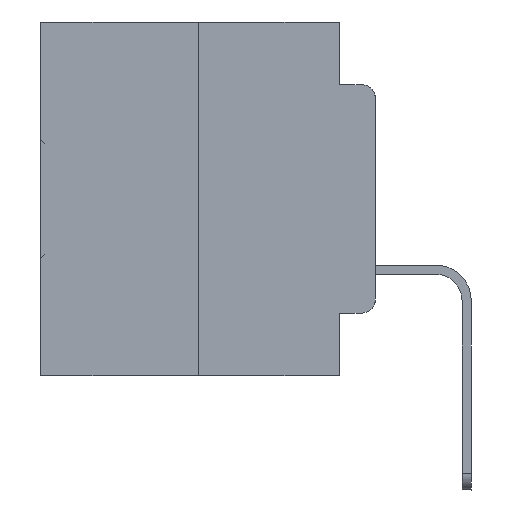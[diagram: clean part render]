
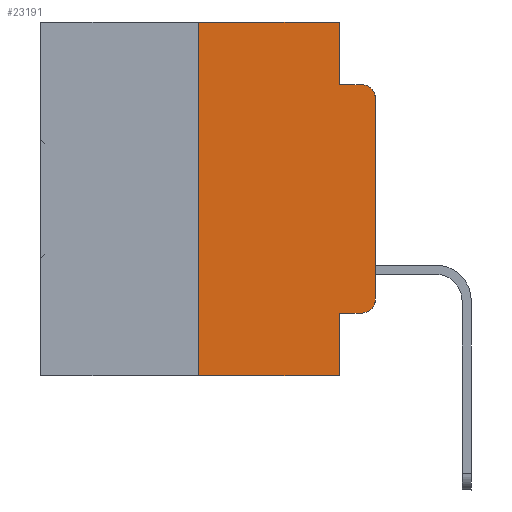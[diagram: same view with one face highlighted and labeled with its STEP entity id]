
A CAD part, left-side view. The second image highlights one B-rep face of the part: STEP entity #23191.
In plain terms, the highlighted planar face has unit normal (-1, 0, 0).
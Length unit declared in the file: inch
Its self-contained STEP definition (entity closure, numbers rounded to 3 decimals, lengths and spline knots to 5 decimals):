
#447 = LINE ( 'NONE', #4120, #23621 ) ;
#589 = EDGE_CURVE ( 'NONE', #5227, #32426, #15324, .T. ) ;
#805 = ORIENTED_EDGE ( 'NONE', *, *, #589, .T. ) ;
#882 = CARTESIAN_POINT ( 'NONE',  ( 0., 0.25, 0. ) ) ;
#2688 = DIRECTION ( 'NONE',  ( 0., 0., -1. ) ) ;
#2972 = FACE_OUTER_BOUND ( 'NONE', #23534, .T. ) ;
#3366 = CARTESIAN_POINT ( 'NONE',  ( 0., 0.02, -0.0885 ) ) ;
#3687 = LINE ( 'NONE', #19408, #24400 ) ;
#3835 = DIRECTION ( 'NONE',  ( 0., -1., 0. ) ) ;
#4120 = CARTESIAN_POINT ( 'NONE',  ( 0., 0.051, 0. ) ) ;
#4148 = CARTESIAN_POINT ( 'NONE',  ( 0., 0.25, -0.5 ) ) ;
#4517 = DIRECTION ( 'NONE',  ( 0., 0., -1. ) ) ;
#4857 = VERTEX_POINT ( 'NONE', #15448 ) ;
#5227 = VERTEX_POINT ( 'NONE', #21931 ) ;
#5275 = DIRECTION ( 'NONE',  ( 0., -1., 0. ) ) ;
#5530 = LINE ( 'NONE', #15710, #31941 ) ;
#6323 = DIRECTION ( 'NONE',  ( 0., 0., -1. ) ) ;
#6393 = ORIENTED_EDGE ( 'NONE', *, *, #30646, .T. ) ;
#6413 = CARTESIAN_POINT ( 'NONE',  ( 0., 0.473, -0.5 ) ) ;
#6609 = DIRECTION ( 'NONE',  ( 0., -1., 0. ) ) ;
#6706 = ORIENTED_EDGE ( 'NONE', *, *, #30181, .T. ) ;
#6930 = DIRECTION ( 'NONE',  ( 0., 0., -1. ) ) ;
#7115 = VERTEX_POINT ( 'NONE', #17934 ) ;
#7246 = ORIENTED_EDGE ( 'NONE', *, *, #20168, .F. ) ;
#7881 = DIRECTION ( 'NONE',  ( 0., 0., 1. ) ) ;
#7894 = DIRECTION ( 'NONE',  ( 1., 0., 0. ) ) ;
#9505 = CIRCLE ( 'NONE', #20482, 0.02 ) ;
#9961 = LINE ( 'NONE', #6413, #16021 ) ;
#10180 = CARTESIAN_POINT ( 'NONE',  ( 0., 0.473, 0. ) ) ;
#11095 = EDGE_CURVE ( 'NONE', #29428, #4857, #15806, .T. ) ;
#12012 = VERTEX_POINT ( 'NONE', #19421 ) ;
#12035 = EDGE_CURVE ( 'NONE', #15611, #32426, #31182, .T. ) ;
#12492 = CARTESIAN_POINT ( 'NONE',  ( 0., 0.25, 0. ) ) ;
#14032 = VECTOR ( 'NONE', #6609, 39.37008 ) ;
#14323 = AXIS2_PLACEMENT_3D ( 'NONE', #28902, #7894, #2688 ) ;
#14869 = CARTESIAN_POINT ( 'NONE',  ( 0., 0., -0.3915 ) ) ;
#14994 = EDGE_CURVE ( 'NONE', #33073, #31567, #9505, .T. ) ;
#15324 = CIRCLE ( 'NONE', #30379, 0.02 ) ;
#15448 = CARTESIAN_POINT ( 'NONE',  ( 0., 0.051, 0. ) ) ;
#15611 = VERTEX_POINT ( 'NONE', #22472 ) ;
#15710 = CARTESIAN_POINT ( 'NONE',  ( 0., 0., 0. ) ) ;
#15806 = LINE ( 'NONE', #10180, #26381 ) ;
#16021 = VECTOR ( 'NONE', #3835, 39.37008 ) ;
#16069 = DIRECTION ( 'NONE',  ( 0., 0., 1. ) ) ;
#16298 = ORIENTED_EDGE ( 'NONE', *, *, #17995, .F. ) ;
#16692 = CARTESIAN_POINT ( 'NONE',  ( 0., 0.02, -0.4115 ) ) ;
#17018 = CARTESIAN_POINT ( 'NONE',  ( 0., 0.051, -0.0885 ) ) ;
#17154 = DIRECTION ( 'NONE',  ( 0., 0., -1. ) ) ;
#17934 = CARTESIAN_POINT ( 'NONE',  ( 0., 0.051, -0.5 ) ) ;
#17995 = EDGE_CURVE ( 'NONE', #30776, #29428, #27841, .T. ) ;
#19408 = CARTESIAN_POINT ( 'NONE',  ( 0., 0.051, 0. ) ) ;
#19421 = CARTESIAN_POINT ( 'NONE',  ( 0., 0.051, -0.4115 ) ) ;
#20168 = EDGE_CURVE ( 'NONE', #4857, #15611, #447, .T. ) ;
#20482 = AXIS2_PLACEMENT_3D ( 'NONE', #32682, #25236, #17154 ) ;
#20683 = EDGE_CURVE ( 'NONE', #12012, #7115, #3687, .T. ) ;
#21197 = PLANE ( 'NONE',  #14323 ) ;
#21327 = VECTOR ( 'NONE', #16069, 39.37008 ) ;
#21869 = CARTESIAN_POINT ( 'NONE',  ( 0., 0.051, -0.4115 ) ) ;
#21931 = CARTESIAN_POINT ( 'NONE',  ( 0., 0., -0.1085 ) ) ;
#22472 = CARTESIAN_POINT ( 'NONE',  ( 0., 0.051, -0.0885 ) ) ;
#22573 = ORIENTED_EDGE ( 'NONE', *, *, #11095, .F. ) ;
#23191 = ADVANCED_FACE ( 'NONE', ( #2972 ), #21197, .F. ) ;
#23534 = EDGE_LOOP ( 'NONE', ( #6706, #805, #30043, #7246, #22573, #16298, #32085, #29604, #6393, #30869 ) ) ;
#23621 = VECTOR ( 'NONE', #6930, 39.37008 ) ;
#24301 = VECTOR ( 'NONE', #27238, 39.37008 ) ;
#24400 = VECTOR ( 'NONE', #6323, 39.37008 ) ;
#25236 = DIRECTION ( 'NONE',  ( -1., 0., 0. ) ) ;
#25530 = CARTESIAN_POINT ( 'NONE',  ( 0., 0.02, -0.1085 ) ) ;
#26381 = VECTOR ( 'NONE', #5275, 39.37008 ) ;
#27238 = DIRECTION ( 'NONE',  ( 0., -1., 0. ) ) ;
#27461 = LINE ( 'NONE', #21869, #14032 ) ;
#27841 = LINE ( 'NONE', #882, #21327 ) ;
#27996 = EDGE_CURVE ( 'NONE', #30776, #7115, #9961, .T. ) ;
#28902 = CARTESIAN_POINT ( 'NONE',  ( 0., 0.473, 0. ) ) ;
#29428 = VERTEX_POINT ( 'NONE', #12492 ) ;
#29604 = ORIENTED_EDGE ( 'NONE', *, *, #20683, .F. ) ;
#30043 = ORIENTED_EDGE ( 'NONE', *, *, #12035, .F. ) ;
#30181 = EDGE_CURVE ( 'NONE', #31567, #5227, #5530, .T. ) ;
#30379 = AXIS2_PLACEMENT_3D ( 'NONE', #25530, #32754, #4517 ) ;
#30646 = EDGE_CURVE ( 'NONE', #12012, #33073, #27461, .T. ) ;
#30776 = VERTEX_POINT ( 'NONE', #4148 ) ;
#30869 = ORIENTED_EDGE ( 'NONE', *, *, #14994, .T. ) ;
#31182 = LINE ( 'NONE', #17018, #24301 ) ;
#31567 = VERTEX_POINT ( 'NONE', #14869 ) ;
#31941 = VECTOR ( 'NONE', #7881, 39.37008 ) ;
#32085 = ORIENTED_EDGE ( 'NONE', *, *, #27996, .T. ) ;
#32426 = VERTEX_POINT ( 'NONE', #3366 ) ;
#32682 = CARTESIAN_POINT ( 'NONE',  ( 0., 0.02, -0.3915 ) ) ;
#32754 = DIRECTION ( 'NONE',  ( -1., 0., 0. ) ) ;
#33073 = VERTEX_POINT ( 'NONE', #16692 ) ;
